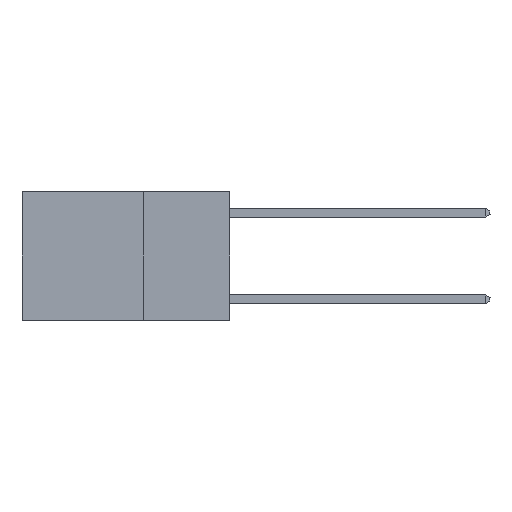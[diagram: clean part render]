
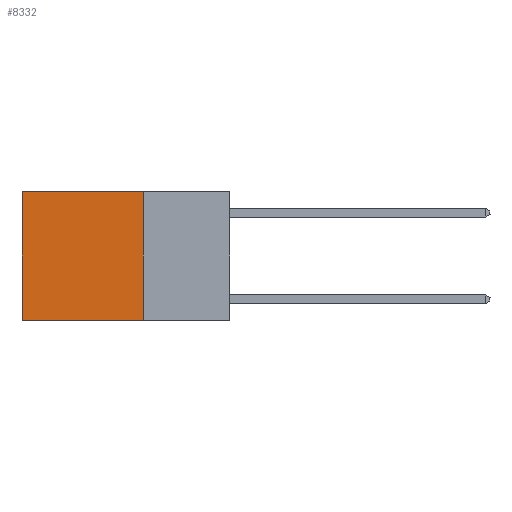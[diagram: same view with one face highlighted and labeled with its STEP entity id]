
A CAD part, left-side view. The second image highlights one B-rep face of the part: STEP entity #8332.
In plain terms, the highlighted planar face has unit normal (-1, 0, 0).
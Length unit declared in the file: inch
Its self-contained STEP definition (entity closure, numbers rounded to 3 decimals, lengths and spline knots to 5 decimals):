
#13 = EDGE_CURVE ( 'NONE', #2001, #15319, #11640, .T. ) ;
#231 = CARTESIAN_POINT ( 'NONE',  ( 0.2625, 0.25, -0.37 ) ) ;
#367 = DIRECTION ( 'NONE',  ( 0., 0., -1. ) ) ;
#1662 = DIRECTION ( 'NONE',  ( 0., 0., -1. ) ) ;
#2001 = VERTEX_POINT ( 'NONE', #10412 ) ;
#2676 = EDGE_LOOP ( 'NONE', ( #5545, #10712, #15355, #13307 ) ) ;
#2961 = CARTESIAN_POINT ( 'NONE',  ( 0.2625, 0.25, 0. ) ) ;
#3153 = VERTEX_POINT ( 'NONE', #11064 ) ;
#3383 = EDGE_CURVE ( 'NONE', #9533, #3153, #15238, .T. ) ;
#3421 = DIRECTION ( 'NONE',  ( 0., 1., 0. ) ) ;
#3987 = CARTESIAN_POINT ( 'NONE',  ( 0.2625, 0.25, 0. ) ) ;
#4260 = CARTESIAN_POINT ( 'NONE',  ( 0.2625, 0.25, 0. ) ) ;
#4813 = VECTOR ( 'NONE', #3421, 39.37008 ) ;
#5545 = ORIENTED_EDGE ( 'NONE', *, *, #15394, .T. ) ;
#7980 = CARTESIAN_POINT ( 'NONE',  ( 0.2625, 0.6, 0. ) ) ;
#8332 = ADVANCED_FACE ( 'NONE', ( #12855 ), #14349, .F. ) ;
#8976 = VECTOR ( 'NONE', #9337, 39.37008 ) ;
#9337 = DIRECTION ( 'NONE',  ( 0., 0., -1. ) ) ;
#9533 = VERTEX_POINT ( 'NONE', #10181 ) ;
#9774 = VECTOR ( 'NONE', #367, 39.37008 ) ;
#10181 = CARTESIAN_POINT ( 'NONE',  ( 0.2625, 0.25, 0. ) ) ;
#10412 = CARTESIAN_POINT ( 'NONE',  ( 0.2625, 0.25, -0.37 ) ) ;
#10453 = VECTOR ( 'NONE', #12763, 39.37008 ) ;
#10712 = ORIENTED_EDGE ( 'NONE', *, *, #13, .F. ) ;
#11064 = CARTESIAN_POINT ( 'NONE',  ( 0.2625, 0.6, 0. ) ) ;
#11640 = LINE ( 'NONE', #231, #4813 ) ;
#12763 = DIRECTION ( 'NONE',  ( 0., 1., 0. ) ) ;
#12855 = FACE_OUTER_BOUND ( 'NONE', #2676, .T. ) ;
#13132 = LINE ( 'NONE', #7980, #9774 ) ;
#13307 = ORIENTED_EDGE ( 'NONE', *, *, #3383, .T. ) ;
#14349 = PLANE ( 'NONE',  #14662 ) ;
#14476 = LINE ( 'NONE', #2961, #8976 ) ;
#14662 = AXIS2_PLACEMENT_3D ( 'NONE', #4260, #15759, #1662 ) ;
#14988 = EDGE_CURVE ( 'NONE', #9533, #2001, #14476, .T. ) ;
#15238 = LINE ( 'NONE', #3987, #10453 ) ;
#15319 = VERTEX_POINT ( 'NONE', #15794 ) ;
#15355 = ORIENTED_EDGE ( 'NONE', *, *, #14988, .F. ) ;
#15394 = EDGE_CURVE ( 'NONE', #3153, #15319, #13132, .T. ) ;
#15759 = DIRECTION ( 'NONE',  ( 1., 0., 0. ) ) ;
#15794 = CARTESIAN_POINT ( 'NONE',  ( 0.2625, 0.6, -0.37 ) ) ;
